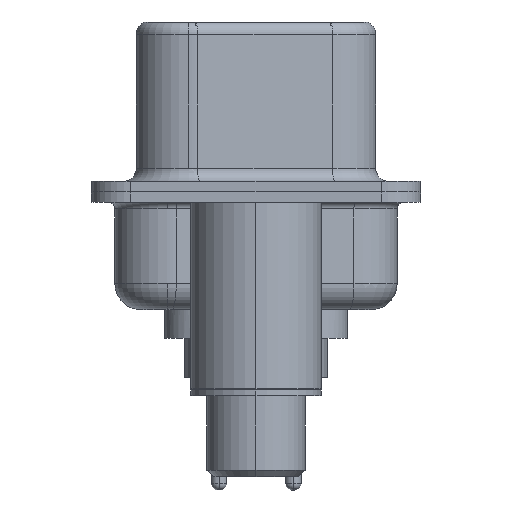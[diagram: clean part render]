
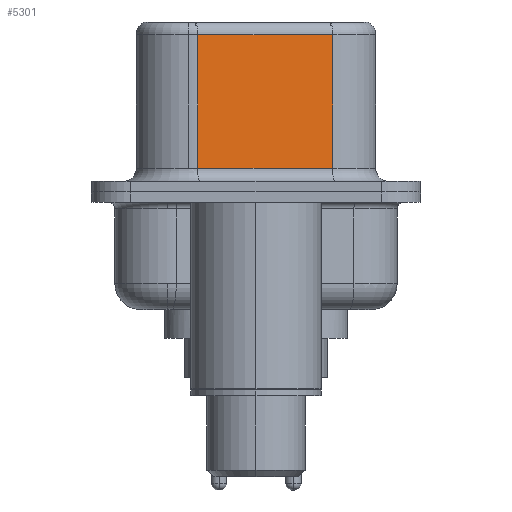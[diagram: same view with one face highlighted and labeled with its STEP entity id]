
A CAD part, left-side view. The second image highlights one B-rep face of the part: STEP entity #5301.
In plain terms, the highlighted planar face has unit normal (-0.985, -0.174, 0).
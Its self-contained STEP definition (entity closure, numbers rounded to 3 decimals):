
#1525 = EDGE_LOOP ( 'NONE', ( #15063, #10715, #11310, #2965 ) ) ;
#1598 = LINE ( 'NONE', #8022, #6433 ) ;
#1909 = LINE ( 'NONE', #8953, #20639 ) ;
#2965 = ORIENTED_EDGE ( 'NONE', *, *, #7607, .T. ) ;
#3083 = EDGE_CURVE ( 'NONE', #12063, #6155, #1909, .T. ) ;
#5049 = DIRECTION ( 'NONE',  ( 0.985, 0.174, 0. ) ) ;
#5301 = ADVANCED_FACE ( 'NONE', ( #20276 ), #13420, .F. ) ;
#5934 = CARTESIAN_POINT ( 'NONE',  ( 3.67, 2.233, 6.02 ) ) ;
#6155 = VERTEX_POINT ( 'NONE', #9237 ) ;
#6433 = VECTOR ( 'NONE', #9837, 1000. ) ;
#6554 = VERTEX_POINT ( 'NONE', #5934 ) ;
#6664 = CARTESIAN_POINT ( 'NONE',  ( 4.58, -2.927, 6.52 ) ) ;
#6952 = VERTEX_POINT ( 'NONE', #10740 ) ;
#7076 = DIRECTION ( 'NONE',  ( -0.174, 0.985, 0. ) ) ;
#7181 = VECTOR ( 'NONE', #19518, 1000. ) ;
#7607 = EDGE_CURVE ( 'NONE', #6952, #6155, #12001, .T. ) ;
#7821 = CARTESIAN_POINT ( 'NONE',  ( 4.58, -2.927, 6.02 ) ) ;
#8022 = CARTESIAN_POINT ( 'NONE',  ( 4.58, -2.927, 6.02 ) ) ;
#8953 = CARTESIAN_POINT ( 'NONE',  ( 4.58, -2.927, 6.52 ) ) ;
#9237 = CARTESIAN_POINT ( 'NONE',  ( 4.58, -2.927, 0.9 ) ) ;
#9837 = DIRECTION ( 'NONE',  ( -0.174, 0.985, 0. ) ) ;
#10715 = ORIENTED_EDGE ( 'NONE', *, *, #17513, .T. ) ;
#10740 = CARTESIAN_POINT ( 'NONE',  ( 3.67, 2.233, 0.9 ) ) ;
#11310 = ORIENTED_EDGE ( 'NONE', *, *, #11404, .T. ) ;
#11404 = EDGE_CURVE ( 'NONE', #6554, #6952, #13405, .T. ) ;
#12001 = LINE ( 'NONE', #19444, #7181 ) ;
#12063 = VERTEX_POINT ( 'NONE', #7821 ) ;
#13405 = LINE ( 'NONE', #16678, #22488 ) ;
#13420 = PLANE ( 'NONE',  #18291 ) ;
#14871 = DIRECTION ( 'NONE',  ( 0., 0., -1. ) ) ;
#15063 = ORIENTED_EDGE ( 'NONE', *, *, #3083, .F. ) ;
#16678 = CARTESIAN_POINT ( 'NONE',  ( 3.67, 2.233, 6.52 ) ) ;
#17513 = EDGE_CURVE ( 'NONE', #12063, #6554, #1598, .T. ) ;
#18291 = AXIS2_PLACEMENT_3D ( 'NONE', #6664, #5049, #7076 ) ;
#19412 = DIRECTION ( 'NONE',  ( 0., 0., -1. ) ) ;
#19444 = CARTESIAN_POINT ( 'NONE',  ( 4.58, -2.927, 0.9 ) ) ;
#19518 = DIRECTION ( 'NONE',  ( 0.174, -0.985, 0. ) ) ;
#20276 = FACE_OUTER_BOUND ( 'NONE', #1525, .T. ) ;
#20639 = VECTOR ( 'NONE', #19412, 1000. ) ;
#22488 = VECTOR ( 'NONE', #14871, 1000. ) ;
